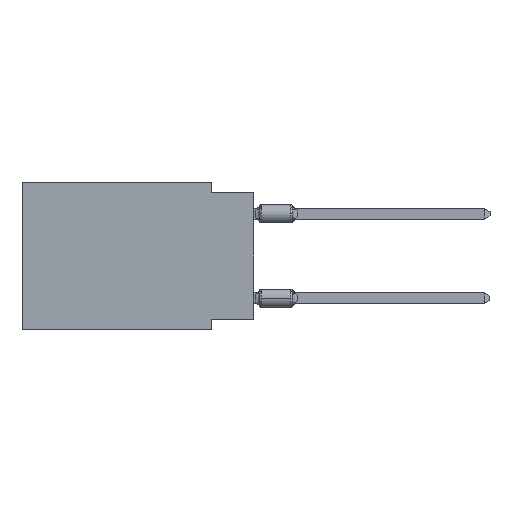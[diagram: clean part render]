
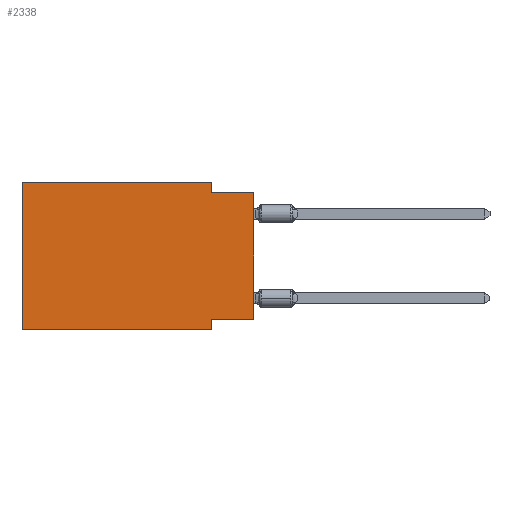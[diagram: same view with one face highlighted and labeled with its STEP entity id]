
A CAD part, left-side view. The second image highlights one B-rep face of the part: STEP entity #2338.
In plain terms, the highlighted planar face has unit normal (-1, 0, 0).
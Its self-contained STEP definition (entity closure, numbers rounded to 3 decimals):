
#13 = CARTESIAN_POINT ( 'NONE',  ( 0., 0., -0.635 ) ) ;
#116 = DIRECTION ( 'NONE',  ( 0., 0., 1. ) ) ;
#1495 = CARTESIAN_POINT ( 'NONE',  ( 0., 2.54, 0. ) ) ;
#1526 = CARTESIAN_POINT ( 'NONE',  ( 0., 0., -8.255 ) ) ;
#1713 = VECTOR ( 'NONE', #12172, 1000. ) ;
#1743 = CARTESIAN_POINT ( 'NONE',  ( 0., 2.54, -0.635 ) ) ;
#1787 = DIRECTION ( 'NONE',  ( 0., -1., 0. ) ) ;
#2338 = ADVANCED_FACE ( 'NONE', ( #27412 ), #32921, .F. ) ;
#3060 = EDGE_CURVE ( 'NONE', #17495, #4831, #23769, .T. ) ;
#3084 = CARTESIAN_POINT ( 'NONE',  ( 0., 13.97, 0. ) ) ;
#3189 = VECTOR ( 'NONE', #4622, 1000. ) ;
#3790 = CARTESIAN_POINT ( 'NONE',  ( 0., 0., -0.635 ) ) ;
#4087 = ORIENTED_EDGE ( 'NONE', *, *, #3060, .T. ) ;
#4109 = CARTESIAN_POINT ( 'NONE',  ( 0., 13.97, -8.89 ) ) ;
#4378 = VERTEX_POINT ( 'NONE', #11183 ) ;
#4412 = CARTESIAN_POINT ( 'NONE',  ( 0., 2.54, -8.89 ) ) ;
#4622 = DIRECTION ( 'NONE',  ( 0., -1., 0. ) ) ;
#4831 = VERTEX_POINT ( 'NONE', #3790 ) ;
#7079 = VERTEX_POINT ( 'NONE', #22045 ) ;
#8231 = DIRECTION ( 'NONE',  ( 1., 0., 0. ) ) ;
#8531 = EDGE_CURVE ( 'NONE', #15144, #7079, #12593, .T. ) ;
#8933 = CARTESIAN_POINT ( 'NONE',  ( 0., 0., -8.255 ) ) ;
#10116 = DIRECTION ( 'NONE',  ( 0., 1., 0. ) ) ;
#10316 = DIRECTION ( 'NONE',  ( 0., 0., 1. ) ) ;
#10740 = DIRECTION ( 'NONE',  ( 0., 0., -1. ) ) ;
#11183 = CARTESIAN_POINT ( 'NONE',  ( 0., 13.97, -8.89 ) ) ;
#12164 = ORIENTED_EDGE ( 'NONE', *, *, #19528, .T. ) ;
#12172 = DIRECTION ( 'NONE',  ( 0., 0., -1. ) ) ;
#12593 = LINE ( 'NONE', #4412, #15281 ) ;
#14053 = VERTEX_POINT ( 'NONE', #1743 ) ;
#14808 = ORIENTED_EDGE ( 'NONE', *, *, #24172, .F. ) ;
#14973 = VECTOR ( 'NONE', #23528, 1000. ) ;
#15144 = VERTEX_POINT ( 'NONE', #30560 ) ;
#15281 = VECTOR ( 'NONE', #28945, 1000. ) ;
#15294 = LINE ( 'NONE', #4109, #28812 ) ;
#15750 = CARTESIAN_POINT ( 'NONE',  ( 0., 0., 0. ) ) ;
#16993 = ORIENTED_EDGE ( 'NONE', *, *, #33191, .F. ) ;
#17495 = VERTEX_POINT ( 'NONE', #1526 ) ;
#17983 = EDGE_CURVE ( 'NONE', #14053, #4831, #24367, .T. ) ;
#18127 = CARTESIAN_POINT ( 'NONE',  ( 0., 13.97, 0. ) ) ;
#18657 = VECTOR ( 'NONE', #10116, 1000. ) ;
#19028 = LINE ( 'NONE', #21695, #14973 ) ;
#19158 = CARTESIAN_POINT ( 'NONE',  ( 0., 2.54, 0. ) ) ;
#19528 = EDGE_CURVE ( 'NONE', #4378, #7079, #15294, .T. ) ;
#20219 = VECTOR ( 'NONE', #116, 1000. ) ;
#20507 = LINE ( 'NONE', #1495, #1713 ) ;
#21695 = CARTESIAN_POINT ( 'NONE',  ( 0., 13.97, 0. ) ) ;
#22042 = EDGE_CURVE ( 'NONE', #17495, #15144, #27935, .T. ) ;
#22045 = CARTESIAN_POINT ( 'NONE',  ( 0., 2.54, -8.89 ) ) ;
#22286 = VERTEX_POINT ( 'NONE', #19158 ) ;
#23528 = DIRECTION ( 'NONE',  ( 0., -1., 0. ) ) ;
#23769 = LINE ( 'NONE', #15750, #20219 ) ;
#23822 = LINE ( 'NONE', #18127, #27485 ) ;
#24172 = EDGE_CURVE ( 'NONE', #22286, #14053, #20507, .T. ) ;
#24367 = LINE ( 'NONE', #13, #3189 ) ;
#25851 = AXIS2_PLACEMENT_3D ( 'NONE', #32401, #8231, #10740 ) ;
#27347 = VERTEX_POINT ( 'NONE', #3084 ) ;
#27412 = FACE_OUTER_BOUND ( 'NONE', #34228, .T. ) ;
#27481 = ORIENTED_EDGE ( 'NONE', *, *, #29943, .F. ) ;
#27485 = VECTOR ( 'NONE', #10316, 1000. ) ;
#27935 = LINE ( 'NONE', #8933, #18657 ) ;
#28812 = VECTOR ( 'NONE', #1787, 1000. ) ;
#28945 = DIRECTION ( 'NONE',  ( 0., 0., -1. ) ) ;
#29943 = EDGE_CURVE ( 'NONE', #27347, #22286, #19028, .T. ) ;
#30490 = ORIENTED_EDGE ( 'NONE', *, *, #17983, .F. ) ;
#30560 = CARTESIAN_POINT ( 'NONE',  ( 0., 2.54, -8.255 ) ) ;
#32401 = CARTESIAN_POINT ( 'NONE',  ( 0., 13.97, 0. ) ) ;
#32921 = PLANE ( 'NONE',  #25851 ) ;
#33191 = EDGE_CURVE ( 'NONE', #4378, #27347, #23822, .T. ) ;
#34228 = EDGE_LOOP ( 'NONE', ( #4087, #30490, #14808, #27481, #16993, #12164, #34416, #34442 ) ) ;
#34416 = ORIENTED_EDGE ( 'NONE', *, *, #8531, .F. ) ;
#34442 = ORIENTED_EDGE ( 'NONE', *, *, #22042, .F. ) ;
